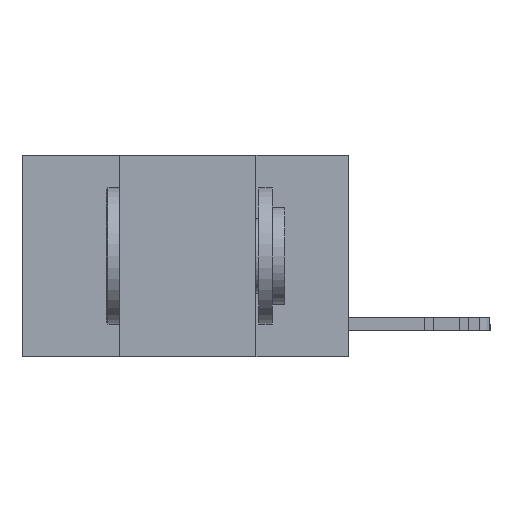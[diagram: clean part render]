
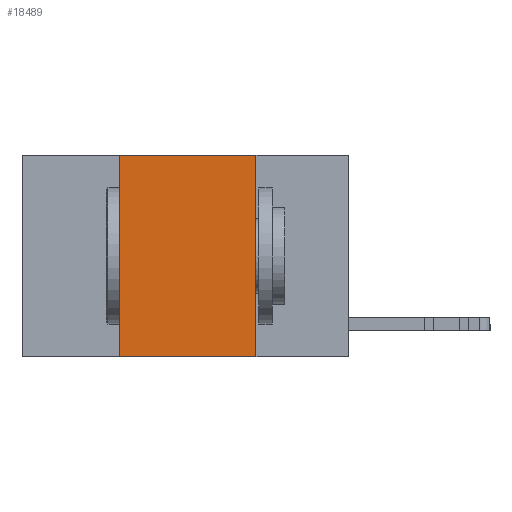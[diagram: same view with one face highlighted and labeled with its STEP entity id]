
A CAD part, left-side view. The second image highlights one B-rep face of the part: STEP entity #18489.
In plain terms, the highlighted planar face has unit normal (-1, 0, 0).
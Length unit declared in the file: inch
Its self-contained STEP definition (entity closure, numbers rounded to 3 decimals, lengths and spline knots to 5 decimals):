
#243 = LINE ( 'NONE', #8566, #4332 ) ;
#776 = CARTESIAN_POINT ( 'NONE',  ( 0., 0.17, -0.37 ) ) ;
#2276 = FACE_OUTER_BOUND ( 'NONE', #5355, .T. ) ;
#2545 = DIRECTION ( 'NONE',  ( 0., 0., 1. ) ) ;
#2932 = LINE ( 'NONE', #11237, #24098 ) ;
#4287 = CARTESIAN_POINT ( 'NONE',  ( 0., 0.6, 0. ) ) ;
#4332 = VECTOR ( 'NONE', #2545, 39.37008 ) ;
#5026 = CARTESIAN_POINT ( 'NONE',  ( 0., 0.17, 0. ) ) ;
#5281 = ORIENTED_EDGE ( 'NONE', *, *, #24276, .F. ) ;
#5355 = EDGE_LOOP ( 'NONE', ( #23247, #5567, #5281, #11664 ) ) ;
#5567 = ORIENTED_EDGE ( 'NONE', *, *, #7952, .F. ) ;
#6201 = CARTESIAN_POINT ( 'NONE',  ( 0., 0.17, 0. ) ) ;
#6430 = PLANE ( 'NONE',  #21059 ) ;
#7952 = EDGE_CURVE ( 'NONE', #15299, #18147, #24393, .T. ) ;
#8549 = DIRECTION ( 'NONE',  ( 0., -1., 0. ) ) ;
#8566 = CARTESIAN_POINT ( 'NONE',  ( 0., 0.42, 0. ) ) ;
#9488 = CARTESIAN_POINT ( 'NONE',  ( 0., 0.42, -0.37 ) ) ;
#10717 = DIRECTION ( 'NONE',  ( 0., 0., -1. ) ) ;
#10766 = EDGE_CURVE ( 'NONE', #18147, #13974, #25762, .T. ) ;
#11142 = DIRECTION ( 'NONE',  ( 1., 0., 0. ) ) ;
#11237 = CARTESIAN_POINT ( 'NONE',  ( 0., 0.6, -0.37 ) ) ;
#11664 = ORIENTED_EDGE ( 'NONE', *, *, #28209, .T. ) ;
#13974 = VERTEX_POINT ( 'NONE', #776 ) ;
#14566 = VERTEX_POINT ( 'NONE', #9488 ) ;
#15299 = VERTEX_POINT ( 'NONE', #16080 ) ;
#16080 = CARTESIAN_POINT ( 'NONE',  ( 0., 0.42, 0. ) ) ;
#18147 = VERTEX_POINT ( 'NONE', #5026 ) ;
#18489 = ADVANCED_FACE ( 'NONE', ( #2276 ), #6430, .F. ) ;
#20633 = VECTOR ( 'NONE', #8549, 39.37008 ) ;
#21059 = AXIS2_PLACEMENT_3D ( 'NONE', #4287, #11142, #10717 ) ;
#21496 = DIRECTION ( 'NONE',  ( 0., 0., -1. ) ) ;
#23247 = ORIENTED_EDGE ( 'NONE', *, *, #10766, .F. ) ;
#24095 = DIRECTION ( 'NONE',  ( 0., -1., 0. ) ) ;
#24098 = VECTOR ( 'NONE', #24095, 39.37008 ) ;
#24276 = EDGE_CURVE ( 'NONE', #14566, #15299, #243, .T. ) ;
#24393 = LINE ( 'NONE', #28119, #20633 ) ;
#25762 = LINE ( 'NONE', #6201, #27112 ) ;
#27112 = VECTOR ( 'NONE', #21496, 39.37008 ) ;
#28119 = CARTESIAN_POINT ( 'NONE',  ( 0., 0.6, 0. ) ) ;
#28209 = EDGE_CURVE ( 'NONE', #14566, #13974, #2932, .T. ) ;
